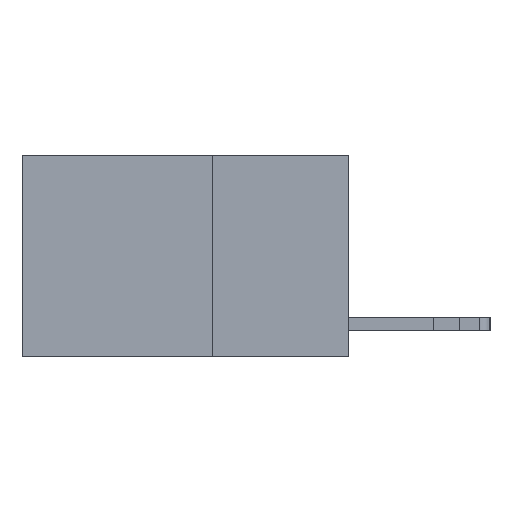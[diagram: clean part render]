
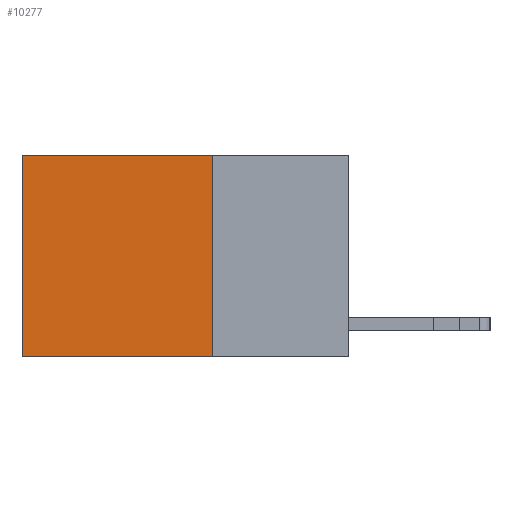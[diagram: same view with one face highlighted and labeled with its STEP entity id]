
A CAD part, left-side view. The second image highlights one B-rep face of the part: STEP entity #10277.
In plain terms, the highlighted planar face has unit normal (-1, 0, 0).
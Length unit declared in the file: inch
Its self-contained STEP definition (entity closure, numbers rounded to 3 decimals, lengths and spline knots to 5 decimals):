
#40 = EDGE_CURVE ( 'NONE', #3623, #18392, #615, .T. ) ;
#615 = LINE ( 'NONE', #2464, #4781 ) ;
#645 = DIRECTION ( 'NONE',  ( 1., 0., 0. ) ) ;
#779 = DIRECTION ( 'NONE',  ( 0., 0., -1. ) ) ;
#910 = CARTESIAN_POINT ( 'NONE',  ( 0.2625, 0.25, 0. ) ) ;
#2366 = DIRECTION ( 'NONE',  ( 0., 0., -1. ) ) ;
#2464 = CARTESIAN_POINT ( 'NONE',  ( 0.2625, 0.25, -0.37 ) ) ;
#2495 = CARTESIAN_POINT ( 'NONE',  ( 0.2625, 0.25, 0. ) ) ;
#3623 = VERTEX_POINT ( 'NONE', #13058 ) ;
#4781 = VECTOR ( 'NONE', #10336, 39.37008 ) ;
#5285 = CARTESIAN_POINT ( 'NONE',  ( 0.2625, 0.25, 0. ) ) ;
#5360 = VECTOR ( 'NONE', #20154, 39.37008 ) ;
#5463 = EDGE_CURVE ( 'NONE', #11968, #3623, #23398, .T. ) ;
#7920 = EDGE_LOOP ( 'NONE', ( #23584, #20502, #18465, #11864 ) ) ;
#8551 = AXIS2_PLACEMENT_3D ( 'NONE', #2495, #645, #19711 ) ;
#8967 = LINE ( 'NONE', #5285, #5360 ) ;
#10277 = ADVANCED_FACE ( 'NONE', ( #13692 ), #17616, .F. ) ;
#10336 = DIRECTION ( 'NONE',  ( 0., 1., 0. ) ) ;
#11864 = ORIENTED_EDGE ( 'NONE', *, *, #14299, .T. ) ;
#11968 = VERTEX_POINT ( 'NONE', #17596 ) ;
#13058 = CARTESIAN_POINT ( 'NONE',  ( 0.2625, 0.25, -0.37 ) ) ;
#13692 = FACE_OUTER_BOUND ( 'NONE', #7920, .T. ) ;
#14299 = EDGE_CURVE ( 'NONE', #11968, #22780, #8967, .T. ) ;
#14800 = CARTESIAN_POINT ( 'NONE',  ( 0.2625, 0.6, -0.37 ) ) ;
#15495 = EDGE_CURVE ( 'NONE', #22780, #18392, #15785, .T. ) ;
#15659 = CARTESIAN_POINT ( 'NONE',  ( 0.2625, 0.6, 0. ) ) ;
#15785 = LINE ( 'NONE', #15659, #18728 ) ;
#17596 = CARTESIAN_POINT ( 'NONE',  ( 0.2625, 0.25, 0. ) ) ;
#17616 = PLANE ( 'NONE',  #8551 ) ;
#18316 = CARTESIAN_POINT ( 'NONE',  ( 0.2625, 0.6, 0. ) ) ;
#18392 = VERTEX_POINT ( 'NONE', #14800 ) ;
#18465 = ORIENTED_EDGE ( 'NONE', *, *, #5463, .F. ) ;
#18728 = VECTOR ( 'NONE', #2366, 39.37008 ) ;
#19711 = DIRECTION ( 'NONE',  ( 0., 0., -1. ) ) ;
#20154 = DIRECTION ( 'NONE',  ( 0., 1., 0. ) ) ;
#20502 = ORIENTED_EDGE ( 'NONE', *, *, #40, .F. ) ;
#21385 = VECTOR ( 'NONE', #779, 39.37008 ) ;
#22780 = VERTEX_POINT ( 'NONE', #18316 ) ;
#23398 = LINE ( 'NONE', #910, #21385 ) ;
#23584 = ORIENTED_EDGE ( 'NONE', *, *, #15495, .T. ) ;
